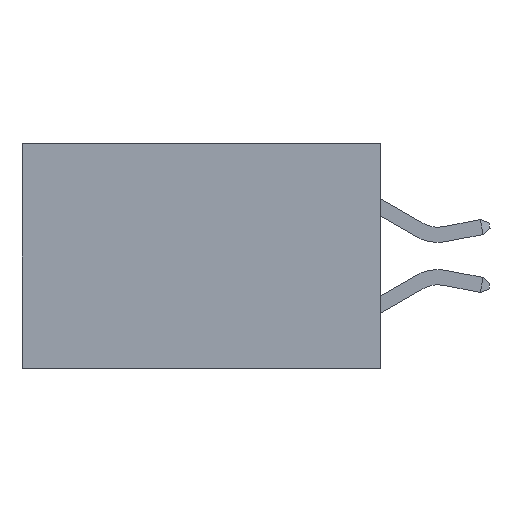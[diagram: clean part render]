
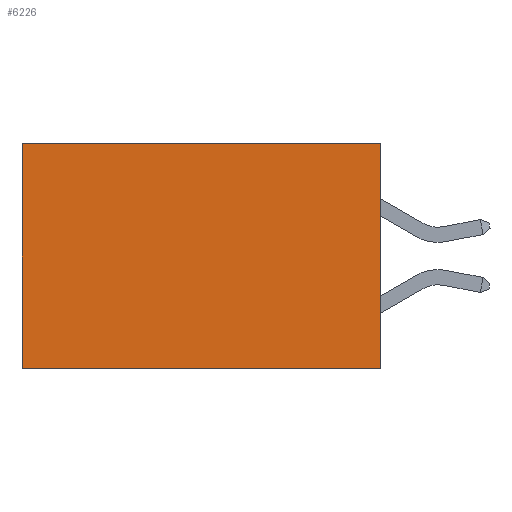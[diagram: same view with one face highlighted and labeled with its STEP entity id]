
A CAD part, left-side view. The second image highlights one B-rep face of the part: STEP entity #6226.
In plain terms, the highlighted planar face has unit normal (-1, 0, 0).
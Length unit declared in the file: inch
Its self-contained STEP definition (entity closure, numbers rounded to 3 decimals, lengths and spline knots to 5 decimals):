
#407 = CARTESIAN_POINT ( 'NONE',  ( 0.277, 0., -0.37 ) ) ;
#1114 = DIRECTION ( 'NONE',  ( 0., 0., -1. ) ) ;
#1287 = EDGE_LOOP ( 'NONE', ( #20786, #20927, #21230, #21421 ) ) ;
#2097 = CARTESIAN_POINT ( 'NONE',  ( 0.277, 0.59, -0.37 ) ) ;
#2954 = CARTESIAN_POINT ( 'NONE',  ( 0.277, 0.59, -0.37 ) ) ;
#3794 = VECTOR ( 'NONE', #9301, 39.37008 ) ;
#3832 = VECTOR ( 'NONE', #1114, 39.37008 ) ;
#4052 = EDGE_CURVE ( 'NONE', #6366, #7160, #10405, .T. ) ;
#4485 = LINE ( 'NONE', #25056, #3832 ) ;
#4604 = FACE_OUTER_BOUND ( 'NONE', #1287, .T. ) ;
#5015 = DIRECTION ( 'NONE',  ( 0., 0., -1. ) ) ;
#6226 = ADVANCED_FACE ( 'NONE', ( #4604 ), #24507, .F. ) ;
#6366 = VERTEX_POINT ( 'NONE', #16923 ) ;
#7160 = VERTEX_POINT ( 'NONE', #23797 ) ;
#9301 = DIRECTION ( 'NONE',  ( 0., 1., 0. ) ) ;
#10405 = LINE ( 'NONE', #12049, #21534 ) ;
#11740 = DIRECTION ( 'NONE',  ( 0., 1., 0. ) ) ;
#12049 = CARTESIAN_POINT ( 'NONE',  ( 0.277, 0., 0. ) ) ;
#14032 = AXIS2_PLACEMENT_3D ( 'NONE', #24478, #24396, #24335 ) ;
#15038 = EDGE_CURVE ( 'NONE', #19581, #23427, #19162, .T. ) ;
#16923 = CARTESIAN_POINT ( 'NONE',  ( 0.277, 0., 0. ) ) ;
#17453 = EDGE_CURVE ( 'NONE', #6366, #19581, #4485, .T. ) ;
#19162 = LINE ( 'NONE', #21144, #3794 ) ;
#19581 = VERTEX_POINT ( 'NONE', #407 ) ;
#20648 = LINE ( 'NONE', #2954, #25287 ) ;
#20786 = ORIENTED_EDGE ( 'NONE', *, *, #24292, .T. ) ;
#20927 = ORIENTED_EDGE ( 'NONE', *, *, #15038, .F. ) ;
#21144 = CARTESIAN_POINT ( 'NONE',  ( 0.277, 0., -0.37 ) ) ;
#21230 = ORIENTED_EDGE ( 'NONE', *, *, #17453, .F. ) ;
#21421 = ORIENTED_EDGE ( 'NONE', *, *, #4052, .T. ) ;
#21534 = VECTOR ( 'NONE', #11740, 39.37008 ) ;
#23427 = VERTEX_POINT ( 'NONE', #2097 ) ;
#23797 = CARTESIAN_POINT ( 'NONE',  ( 0.277, 0.59, 0. ) ) ;
#24292 = EDGE_CURVE ( 'NONE', #7160, #23427, #20648, .T. ) ;
#24335 = DIRECTION ( 'NONE',  ( 0., 0., -1. ) ) ;
#24396 = DIRECTION ( 'NONE',  ( 1., 0., 0. ) ) ;
#24478 = CARTESIAN_POINT ( 'NONE',  ( 0.277, 0., -0.37 ) ) ;
#24507 = PLANE ( 'NONE',  #14032 ) ;
#25056 = CARTESIAN_POINT ( 'NONE',  ( 0.277, 0., -0.37 ) ) ;
#25287 = VECTOR ( 'NONE', #5015, 39.37008 ) ;
